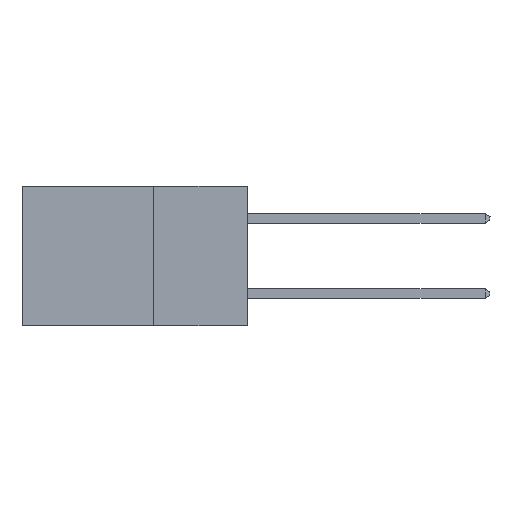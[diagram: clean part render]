
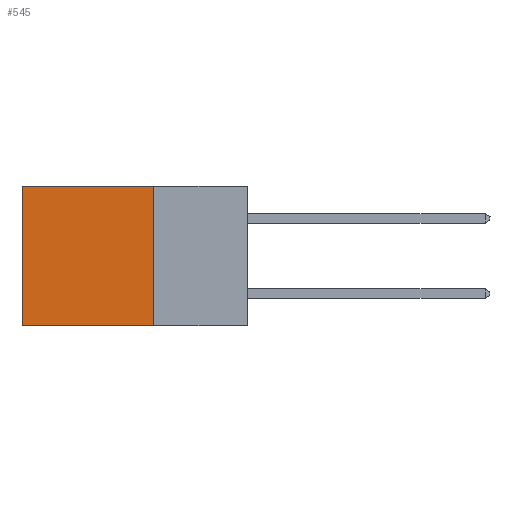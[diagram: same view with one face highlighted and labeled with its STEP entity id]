
A CAD part, left-side view. The second image highlights one B-rep face of the part: STEP entity #545.
In plain terms, the highlighted planar face has unit normal (-1, 0, 0).
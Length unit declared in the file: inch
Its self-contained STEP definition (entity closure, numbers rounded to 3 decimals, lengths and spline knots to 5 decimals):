
#173 = VERTEX_POINT ( 'NONE', #16387 ) ;
#545 = ADVANCED_FACE ( 'NONE', ( #5008 ), #13748, .F. ) ;
#1356 = CARTESIAN_POINT ( 'NONE',  ( 0.298, 0.6, 0. ) ) ;
#1520 = LINE ( 'NONE', #12969, #10428 ) ;
#2023 = DIRECTION ( 'NONE',  ( 0., 1., 0. ) ) ;
#2112 = AXIS2_PLACEMENT_3D ( 'NONE', #4456, #4525, #2790 ) ;
#2723 = ORIENTED_EDGE ( 'NONE', *, *, #18950, .T. ) ;
#2790 = DIRECTION ( 'NONE',  ( 0., 0., -1. ) ) ;
#3331 = VECTOR ( 'NONE', #5535, 39.37008 ) ;
#4456 = CARTESIAN_POINT ( 'NONE',  ( 0.298, 0.25, 0. ) ) ;
#4525 = DIRECTION ( 'NONE',  ( 1., 0., 0. ) ) ;
#5008 = FACE_OUTER_BOUND ( 'NONE', #5764, .T. ) ;
#5535 = DIRECTION ( 'NONE',  ( 0., 1., 0. ) ) ;
#5764 = EDGE_LOOP ( 'NONE', ( #2723, #13927, #19143, #13731 ) ) ;
#5859 = VERTEX_POINT ( 'NONE', #6950 ) ;
#6417 = LINE ( 'NONE', #18174, #12468 ) ;
#6950 = CARTESIAN_POINT ( 'NONE',  ( 0.298, 0.6, -0.37 ) ) ;
#9821 = CARTESIAN_POINT ( 'NONE',  ( 0.298, 0.6, 0. ) ) ;
#10428 = VECTOR ( 'NONE', #2023, 39.37008 ) ;
#12259 = VECTOR ( 'NONE', #21605, 39.37008 ) ;
#12468 = VECTOR ( 'NONE', #12772, 39.37008 ) ;
#12772 = DIRECTION ( 'NONE',  ( 0., 0., -1. ) ) ;
#12969 = CARTESIAN_POINT ( 'NONE',  ( 0.298, 0.25, -0.37 ) ) ;
#13731 = ORIENTED_EDGE ( 'NONE', *, *, #19219, .T. ) ;
#13748 = PLANE ( 'NONE',  #2112 ) ;
#13853 = EDGE_CURVE ( 'NONE', #173, #16652, #6417, .T. ) ;
#13927 = ORIENTED_EDGE ( 'NONE', *, *, #22103, .F. ) ;
#14520 = LINE ( 'NONE', #1356, #12259 ) ;
#16387 = CARTESIAN_POINT ( 'NONE',  ( 0.298, 0.25, 0. ) ) ;
#16534 = CARTESIAN_POINT ( 'NONE',  ( 0.298, 0.25, -0.37 ) ) ;
#16652 = VERTEX_POINT ( 'NONE', #16534 ) ;
#17914 = LINE ( 'NONE', #20339, #3331 ) ;
#18174 = CARTESIAN_POINT ( 'NONE',  ( 0.298, 0.25, 0. ) ) ;
#18950 = EDGE_CURVE ( 'NONE', #19275, #5859, #14520, .T. ) ;
#19143 = ORIENTED_EDGE ( 'NONE', *, *, #13853, .F. ) ;
#19219 = EDGE_CURVE ( 'NONE', #173, #19275, #17914, .T. ) ;
#19275 = VERTEX_POINT ( 'NONE', #9821 ) ;
#20339 = CARTESIAN_POINT ( 'NONE',  ( 0.298, 0.25, 0. ) ) ;
#21605 = DIRECTION ( 'NONE',  ( 0., 0., -1. ) ) ;
#22103 = EDGE_CURVE ( 'NONE', #16652, #5859, #1520, .T. ) ;
